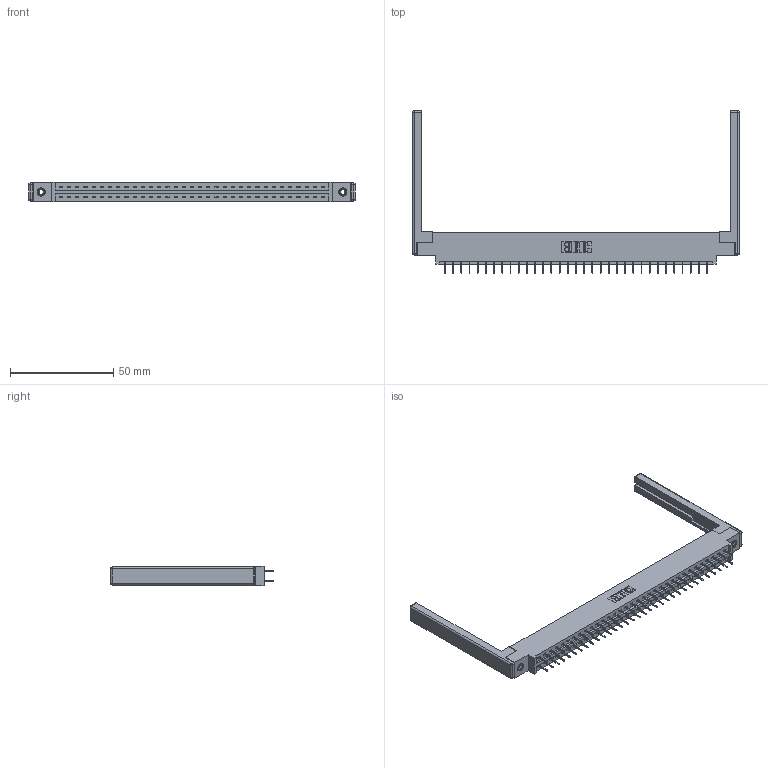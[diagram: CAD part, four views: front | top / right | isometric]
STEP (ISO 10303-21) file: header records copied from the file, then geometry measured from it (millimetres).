
FILE_DESCRIPTION (( 'STEP AP203' ), '1' );
FILE_NAME ('337-066-524-868.STEP', '2019-10-12T00:51:50', ( '' ), ( '' ), 'SwSTEP 2.0', 'SolidWorks 2016', '' );
FILE_SCHEMA (( 'CONFIG_CONTROL_DESIGN' ));
Length unit declared in the file: inch
Products named in the file (5): 345-292-001_345-293-124; 345-250-001_345-250-001-102; 337-066-524-868; 307-220-068; 337 Part_0.170 Offset - 0.156 Dia-TI
Assembly tree (71 placements, depth 2):
  337-066-524-868
    337 Part_0.170 Offset - 0.156 Dia-TI
    345-292-001_345-293-124  x66
    345-250-001_345-250-001-102  x2
    307-220-068  x2
Bounding box: 158.19 x 78.75 x 9.4 mm (x, y, z)
Volume: 20719.1 mm3; surface area: 22211.3 mm2
Topology: 71 solids, 71 shells, 4100 faces, 11603 edges, 7450 vertices
Faces by surface type: plane 3066, cylinder 1010, cone 12, sphere 8, torus 4
Entity records: 29716 total; most frequent: CARTESIAN_POINT 4979, ORIENTED_EDGE 4904, DIRECTION 4322, EDGE_CURVE 2452, VECTOR 2278, LINE 2278, VERTEX_POINT 1622, AXIS2_PLACEMENT_3D 1022
